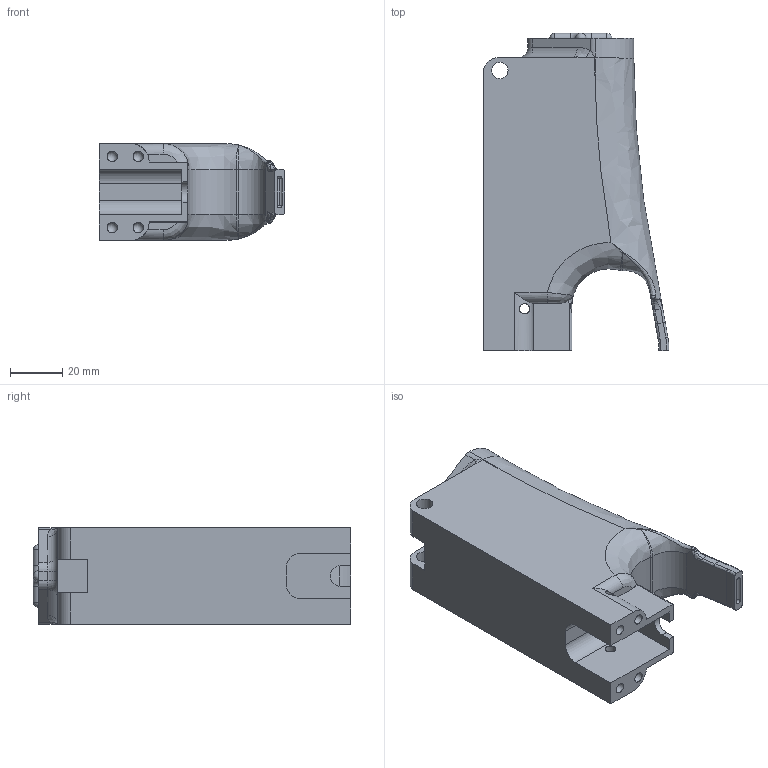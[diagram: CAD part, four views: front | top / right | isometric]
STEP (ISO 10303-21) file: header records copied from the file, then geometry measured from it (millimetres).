
FILE_DESCRIPTION (( 'STEP AP214' ), '1' );
FILE_NAME ('Atlas_SSR_Receiver_Front_V2.step', '2016-01-25T18:17:06', ( 'WarFairy' ), ( '' ), 'SwSTEP 2.0', 'SolidWorks 2015', '' );
FILE_SCHEMA (( 'AUTOMOTIVE_DESIGN' ));
Length unit declared in the file: millimetre
Products named in the file (1): Atlas_SSR_Receiver_Front_V2
Bounding box: 71.28 x 122.01 x 37.13 mm (x, y, z)
Volume: 205010.6 mm3; surface area: 27507 mm2
Topology: 1 solids, 1 shells, 155 faces, 422 edges, 253 vertices
Faces by surface type: bspline 48, cylinder 48, plane 39, torus 10, sphere 10
Full cylindrical faces by diameter (mm): 3.969 x2, 6.375 x2
Entity records: 7773 total; most frequent: CARTESIAN_POINT 4400, ORIENTED_EDGE 774, DIRECTION 581, EDGE_CURVE 387, VERTEX_POINT 244, AXIS2_PLACEMENT_3D 219, EDGE_LOOP 173, FACE_OUTER_BOUND 159
